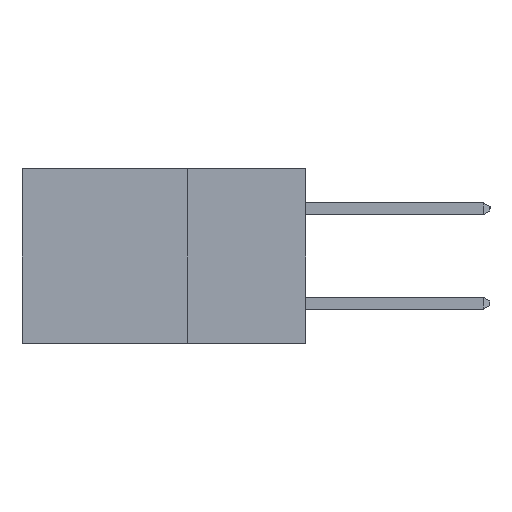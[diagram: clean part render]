
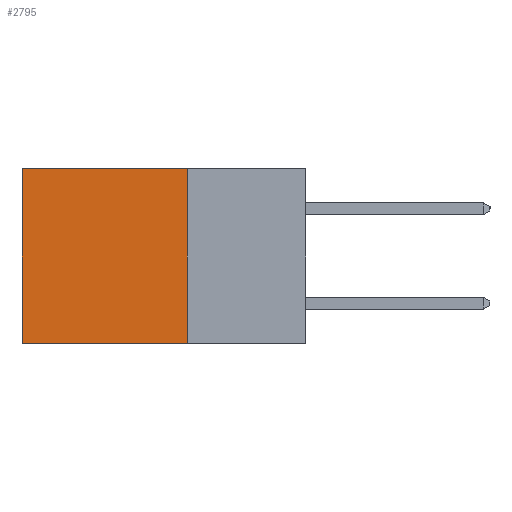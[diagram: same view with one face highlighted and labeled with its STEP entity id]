
A CAD part, left-side view. The second image highlights one B-rep face of the part: STEP entity #2795.
In plain terms, the highlighted planar face has unit normal (-1, 0, 0).
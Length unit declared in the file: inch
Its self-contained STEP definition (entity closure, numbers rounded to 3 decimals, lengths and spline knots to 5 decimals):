
#590 = PLANE ( 'NONE',  #8419 ) ;
#959 = EDGE_CURVE ( 'NONE', #11330, #9918, #1924, .T. ) ;
#1754 = CARTESIAN_POINT ( 'NONE',  ( 0.2615, 0.25, 0. ) ) ;
#1924 = LINE ( 'NONE', #13700, #10021 ) ;
#2364 = ORIENTED_EDGE ( 'NONE', *, *, #13376, .F. ) ;
#2795 = ADVANCED_FACE ( 'NONE', ( #10017 ), #590, .F. ) ;
#3213 = DIRECTION ( 'NONE',  ( 0., 0., -1. ) ) ;
#4308 = DIRECTION ( 'NONE',  ( 1., 0., 0. ) ) ;
#5266 = LINE ( 'NONE', #12320, #11604 ) ;
#5598 = VECTOR ( 'NONE', #7673, 39.37008 ) ;
#5776 = CARTESIAN_POINT ( 'NONE',  ( 0.2615, 0.6, 0. ) ) ;
#6601 = VECTOR ( 'NONE', #3213, 39.37008 ) ;
#7427 = VERTEX_POINT ( 'NONE', #5776 ) ;
#7673 = DIRECTION ( 'NONE',  ( 0., 1., 0. ) ) ;
#7824 = VERTEX_POINT ( 'NONE', #14170 ) ;
#8110 = CARTESIAN_POINT ( 'NONE',  ( 0.2615, 0.25, -0.37 ) ) ;
#8419 = AXIS2_PLACEMENT_3D ( 'NONE', #11428, #4308, #8851 ) ;
#8851 = DIRECTION ( 'NONE',  ( 0., 0., -1. ) ) ;
#8857 = LINE ( 'NONE', #1754, #5598 ) ;
#9918 = VERTEX_POINT ( 'NONE', #13776 ) ;
#10017 = FACE_OUTER_BOUND ( 'NONE', #10366, .T. ) ;
#10021 = VECTOR ( 'NONE', #12617, 39.37008 ) ;
#10047 = DIRECTION ( 'NONE',  ( 0., 0., -1. ) ) ;
#10366 = EDGE_LOOP ( 'NONE', ( #14700, #13339, #2364, #11890 ) ) ;
#11330 = VERTEX_POINT ( 'NONE', #13853 ) ;
#11428 = CARTESIAN_POINT ( 'NONE',  ( 0.2615, 0.25, -0.37 ) ) ;
#11604 = VECTOR ( 'NONE', #10047, 39.37008 ) ;
#11890 = ORIENTED_EDGE ( 'NONE', *, *, #14471, .T. ) ;
#12320 = CARTESIAN_POINT ( 'NONE',  ( 0.2615, 0.6, -0.37 ) ) ;
#12617 = DIRECTION ( 'NONE',  ( 0., 1., 0. ) ) ;
#12711 = EDGE_CURVE ( 'NONE', #7427, #9918, #5266, .T. ) ;
#13339 = ORIENTED_EDGE ( 'NONE', *, *, #959, .F. ) ;
#13376 = EDGE_CURVE ( 'NONE', #7824, #11330, #15066, .T. ) ;
#13700 = CARTESIAN_POINT ( 'NONE',  ( 0.2615, 0.25, -0.37 ) ) ;
#13776 = CARTESIAN_POINT ( 'NONE',  ( 0.2615, 0.6, -0.37 ) ) ;
#13853 = CARTESIAN_POINT ( 'NONE',  ( 0.2615, 0.25, -0.37 ) ) ;
#14170 = CARTESIAN_POINT ( 'NONE',  ( 0.2615, 0.25, 0. ) ) ;
#14471 = EDGE_CURVE ( 'NONE', #7824, #7427, #8857, .T. ) ;
#14700 = ORIENTED_EDGE ( 'NONE', *, *, #12711, .T. ) ;
#15066 = LINE ( 'NONE', #8110, #6601 ) ;
